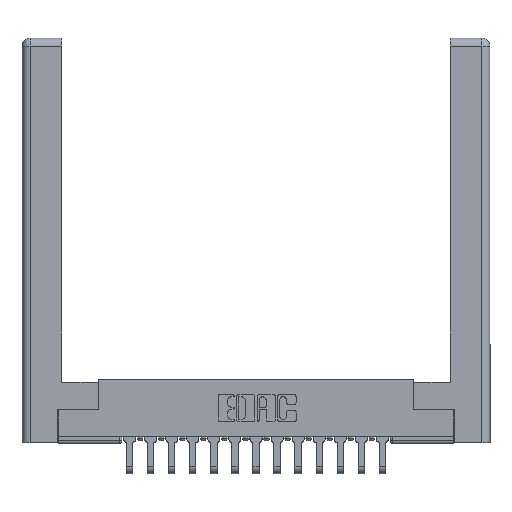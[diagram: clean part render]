
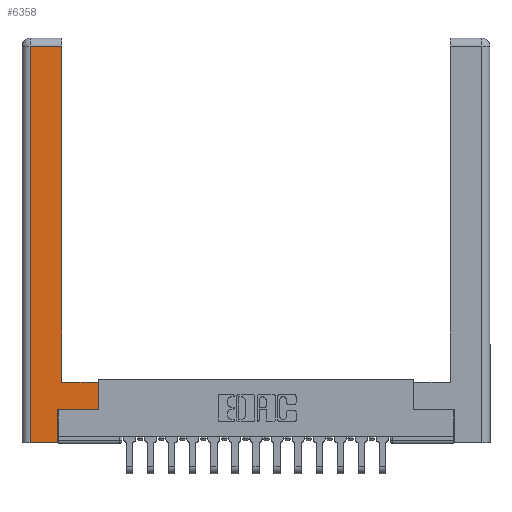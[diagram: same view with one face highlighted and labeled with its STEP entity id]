
A CAD part, top view. The second image highlights one B-rep face of the part: STEP entity #6358.
In plain terms, the highlighted planar face has unit normal (0, 0, 1).
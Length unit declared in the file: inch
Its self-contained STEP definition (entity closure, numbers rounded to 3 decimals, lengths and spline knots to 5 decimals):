
#490 = DIRECTION ( 'NONE',  ( 0., -1., 0. ) ) ;
#523 = CARTESIAN_POINT ( 'NONE',  ( 0.295, 0.45, 0. ) ) ;
#930 = VECTOR ( 'NONE', #15637, 39.37008 ) ;
#1019 = EDGE_CURVE ( 'NONE', #8886, #5986, #15055, .T. ) ;
#1515 = ORIENTED_EDGE ( 'NONE', *, *, #1019, .T. ) ;
#1524 = VECTOR ( 'NONE', #10677, 39.37008 ) ;
#1591 = CARTESIAN_POINT ( 'NONE',  ( 0.565, 0.245, 0. ) ) ;
#1850 = LINE ( 'NONE', #3695, #8762 ) ;
#1889 = CARTESIAN_POINT ( 'NONE',  ( 0.295, 0.45, 0. ) ) ;
#1937 = CARTESIAN_POINT ( 'NONE',  ( 0.265, 0., 0. ) ) ;
#2161 = CARTESIAN_POINT ( 'NONE',  ( 0.265, 0.245, 0. ) ) ;
#2496 = FACE_OUTER_BOUND ( 'NONE', #4234, .T. ) ;
#3027 = VERTEX_POINT ( 'NONE', #9617 ) ;
#3085 = CARTESIAN_POINT ( 'NONE',  ( 0.0615, 2.94, 0. ) ) ;
#3370 = LINE ( 'NONE', #3085, #9084 ) ;
#3400 = LINE ( 'NONE', #1937, #4083 ) ;
#3657 = VECTOR ( 'NONE', #7641, 39.37008 ) ;
#3695 = CARTESIAN_POINT ( 'NONE',  ( 0.0615, 0., 0. ) ) ;
#4083 = VECTOR ( 'NONE', #6414, 39.37008 ) ;
#4162 = CARTESIAN_POINT ( 'NONE',  ( 0.265, 0.245, 0. ) ) ;
#4234 = EDGE_LOOP ( 'NONE', ( #9899, #12219, #10300, #4840, #6348, #10973, #1515, #11521 ) ) ;
#4275 = CARTESIAN_POINT ( 'NONE',  ( 0.565, 0.45, 0. ) ) ;
#4392 = EDGE_CURVE ( 'NONE', #9047, #17036, #3370, .T. ) ;
#4840 = ORIENTED_EDGE ( 'NONE', *, *, #5688, .T. ) ;
#5688 = EDGE_CURVE ( 'NONE', #10539, #3027, #3400, .T. ) ;
#5811 = DIRECTION ( 'NONE',  ( 0., 1., 0. ) ) ;
#5986 = VERTEX_POINT ( 'NONE', #4275 ) ;
#6186 = CARTESIAN_POINT ( 'NONE',  ( 0.565, 0.45, 0. ) ) ;
#6326 = CARTESIAN_POINT ( 'NONE',  ( 0.0615, 0., 0. ) ) ;
#6348 = ORIENTED_EDGE ( 'NONE', *, *, #18230, .T. ) ;
#6358 = ADVANCED_FACE ( 'NONE', ( #2496 ), #8452, .F. ) ;
#6414 = DIRECTION ( 'NONE',  ( 1., 0., 0. ) ) ;
#6565 = DIRECTION ( 'NONE',  ( -1., 0., 0. ) ) ;
#7641 = DIRECTION ( 'NONE',  ( 0., 1., 0. ) ) ;
#7648 = DIRECTION ( 'NONE',  ( -1., 0., 0. ) ) ;
#8058 = CARTESIAN_POINT ( 'NONE',  ( 0.295, 3., 0. ) ) ;
#8254 = LINE ( 'NONE', #8058, #930 ) ;
#8452 = PLANE ( 'NONE',  #12198 ) ;
#8762 = VECTOR ( 'NONE', #490, 39.37008 ) ;
#8819 = DIRECTION ( 'NONE',  ( -1., 0., 0. ) ) ;
#8886 = VERTEX_POINT ( 'NONE', #15565 ) ;
#9047 = VERTEX_POINT ( 'NONE', #13035 ) ;
#9084 = VECTOR ( 'NONE', #7648, 39.37008 ) ;
#9617 = CARTESIAN_POINT ( 'NONE',  ( 0.265, 0., 0. ) ) ;
#9696 = LINE ( 'NONE', #1889, #16682 ) ;
#9899 = ORIENTED_EDGE ( 'NONE', *, *, #18379, .T. ) ;
#10116 = EDGE_CURVE ( 'NONE', #5986, #10204, #9696, .T. ) ;
#10204 = VERTEX_POINT ( 'NONE', #523 ) ;
#10300 = ORIENTED_EDGE ( 'NONE', *, *, #13792, .T. ) ;
#10385 = CARTESIAN_POINT ( 'NONE',  ( 0., 0., 0. ) ) ;
#10539 = VERTEX_POINT ( 'NONE', #6326 ) ;
#10585 = VECTOR ( 'NONE', #5811, 39.37008 ) ;
#10677 = DIRECTION ( 'NONE',  ( 1., 0., 0. ) ) ;
#10973 = ORIENTED_EDGE ( 'NONE', *, *, #17369, .T. ) ;
#11521 = ORIENTED_EDGE ( 'NONE', *, *, #10116, .T. ) ;
#12198 = AXIS2_PLACEMENT_3D ( 'NONE', #10385, #17862, #8819 ) ;
#12219 = ORIENTED_EDGE ( 'NONE', *, *, #4392, .T. ) ;
#12258 = CARTESIAN_POINT ( 'NONE',  ( 0.0615, 2.94, 0. ) ) ;
#13035 = CARTESIAN_POINT ( 'NONE',  ( 0.295, 2.94, 0. ) ) ;
#13308 = VERTEX_POINT ( 'NONE', #2161 ) ;
#13792 = EDGE_CURVE ( 'NONE', #17036, #10539, #1850, .T. ) ;
#15055 = LINE ( 'NONE', #6186, #3657 ) ;
#15565 = CARTESIAN_POINT ( 'NONE',  ( 0.565, 0.245, 0. ) ) ;
#15637 = DIRECTION ( 'NONE',  ( 0., 1., 0. ) ) ;
#16201 = LINE ( 'NONE', #1591, #1524 ) ;
#16682 = VECTOR ( 'NONE', #6565, 39.37008 ) ;
#17036 = VERTEX_POINT ( 'NONE', #12258 ) ;
#17369 = EDGE_CURVE ( 'NONE', #13308, #8886, #16201, .T. ) ;
#17862 = DIRECTION ( 'NONE',  ( 0., 0., -1. ) ) ;
#18230 = EDGE_CURVE ( 'NONE', #3027, #13308, #19159, .T. ) ;
#18379 = EDGE_CURVE ( 'NONE', #10204, #9047, #8254, .T. ) ;
#19159 = LINE ( 'NONE', #4162, #10585 ) ;
